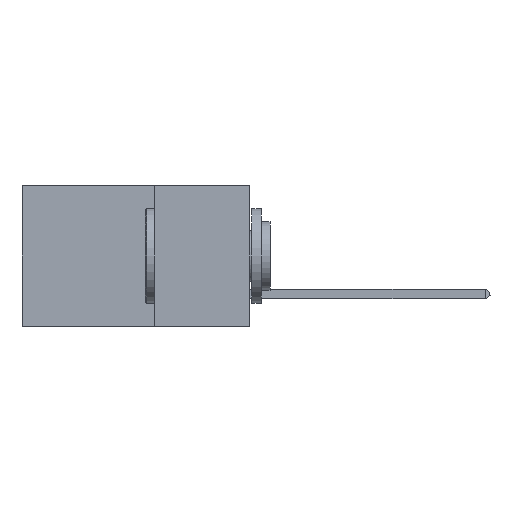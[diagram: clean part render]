
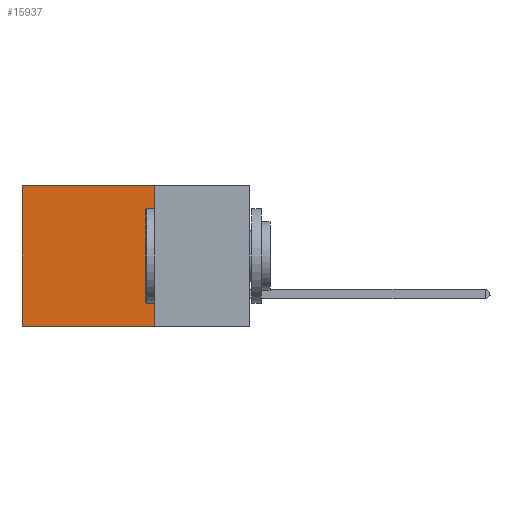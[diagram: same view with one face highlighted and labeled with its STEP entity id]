
A CAD part, left-side view. The second image highlights one B-rep face of the part: STEP entity #15937.
In plain terms, the highlighted planar face has unit normal (-1, 0, 0).
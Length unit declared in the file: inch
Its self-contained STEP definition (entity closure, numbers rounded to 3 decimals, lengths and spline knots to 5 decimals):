
#361 = CARTESIAN_POINT ( 'NONE',  ( 0.2875, 0.25, 0. ) ) ;
#652 = CARTESIAN_POINT ( 'NONE',  ( 0.2875, 0.6, 0. ) ) ;
#768 = CARTESIAN_POINT ( 'NONE',  ( 0.2875, 0.25, 0. ) ) ;
#791 = LINE ( 'NONE', #768, #12702 ) ;
#1982 = VECTOR ( 'NONE', #21713, 39.37008 ) ;
#2363 = CARTESIAN_POINT ( 'NONE',  ( 0.2875, 0.25, 0. ) ) ;
#2825 = LINE ( 'NONE', #361, #1982 ) ;
#4571 = CARTESIAN_POINT ( 'NONE',  ( 0.2875, 0.25, 0. ) ) ;
#6250 = ORIENTED_EDGE ( 'NONE', *, *, #14458, .F. ) ;
#6474 = CARTESIAN_POINT ( 'NONE',  ( 0.2875, 0.25, -0.37 ) ) ;
#6622 = PLANE ( 'NONE',  #12633 ) ;
#6864 = VERTEX_POINT ( 'NONE', #2363 ) ;
#8314 = DIRECTION ( 'NONE',  ( 0., 0., -1. ) ) ;
#8722 = VECTOR ( 'NONE', #15428, 39.37008 ) ;
#9402 = EDGE_CURVE ( 'NONE', #6864, #13955, #791, .T. ) ;
#11877 = VECTOR ( 'NONE', #22079, 39.37008 ) ;
#12633 = AXIS2_PLACEMENT_3D ( 'NONE', #4571, #20563, #22453 ) ;
#12702 = VECTOR ( 'NONE', #8314, 39.37008 ) ;
#12812 = ORIENTED_EDGE ( 'NONE', *, *, #9402, .F. ) ;
#13048 = VERTEX_POINT ( 'NONE', #17150 ) ;
#13955 = VERTEX_POINT ( 'NONE', #17768 ) ;
#13963 = ORIENTED_EDGE ( 'NONE', *, *, #19908, .T. ) ;
#14458 = EDGE_CURVE ( 'NONE', #13955, #13048, #22892, .T. ) ;
#15428 = DIRECTION ( 'NONE',  ( 0., 1., 0. ) ) ;
#15937 = ADVANCED_FACE ( 'NONE', ( #19430 ), #6622, .F. ) ;
#17150 = CARTESIAN_POINT ( 'NONE',  ( 0.2875, 0.6, -0.37 ) ) ;
#17410 = LINE ( 'NONE', #18792, #11877 ) ;
#17768 = CARTESIAN_POINT ( 'NONE',  ( 0.2875, 0.25, -0.37 ) ) ;
#18792 = CARTESIAN_POINT ( 'NONE',  ( 0.2875, 0.6, 0. ) ) ;
#19430 = FACE_OUTER_BOUND ( 'NONE', #22492, .T. ) ;
#19908 = EDGE_CURVE ( 'NONE', #6864, #21472, #2825, .T. ) ;
#20563 = DIRECTION ( 'NONE',  ( 1., 0., 0. ) ) ;
#21472 = VERTEX_POINT ( 'NONE', #652 ) ;
#21615 = EDGE_CURVE ( 'NONE', #21472, #13048, #17410, .T. ) ;
#21695 = ORIENTED_EDGE ( 'NONE', *, *, #21615, .T. ) ;
#21713 = DIRECTION ( 'NONE',  ( 0., 1., 0. ) ) ;
#22079 = DIRECTION ( 'NONE',  ( 0., 0., -1. ) ) ;
#22453 = DIRECTION ( 'NONE',  ( 0., 0., -1. ) ) ;
#22492 = EDGE_LOOP ( 'NONE', ( #21695, #6250, #12812, #13963 ) ) ;
#22892 = LINE ( 'NONE', #6474, #8722 ) ;
